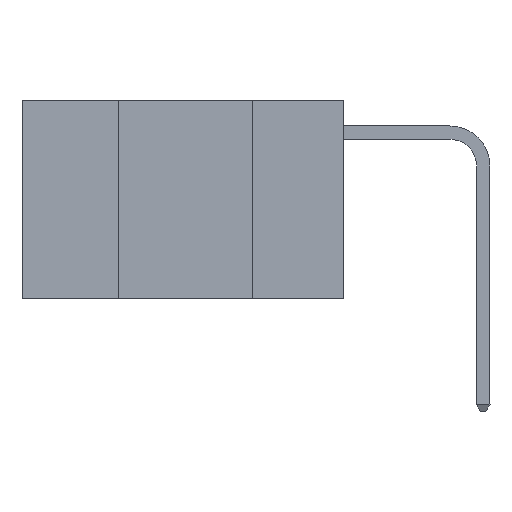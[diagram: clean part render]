
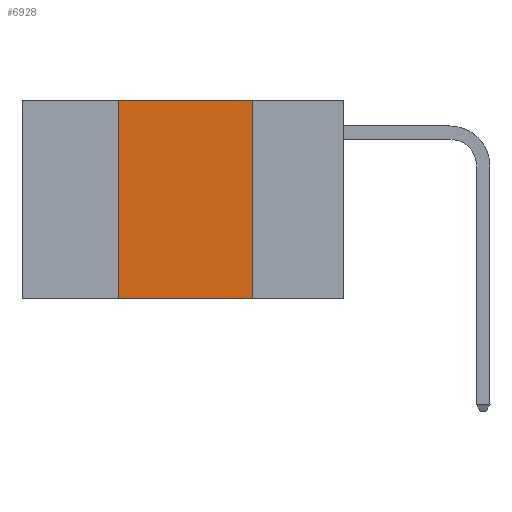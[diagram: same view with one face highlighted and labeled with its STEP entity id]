
A CAD part, left-side view. The second image highlights one B-rep face of the part: STEP entity #6928.
In plain terms, the highlighted planar face has unit normal (-1, 0, 0).
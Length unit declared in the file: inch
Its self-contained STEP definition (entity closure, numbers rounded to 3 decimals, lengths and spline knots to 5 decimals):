
#1199 = ORIENTED_EDGE ( 'NONE', *, *, #21920, .F. ) ;
#1402 = ORIENTED_EDGE ( 'NONE', *, *, #5971, .F. ) ;
#1460 = ORIENTED_EDGE ( 'NONE', *, *, #9302, .F. ) ;
#2199 = ORIENTED_EDGE ( 'NONE', *, *, #6922, .T. ) ;
#3097 = VECTOR ( 'NONE', #21161, 39.37008 ) ;
#3577 = LINE ( 'NONE', #10328, #21398 ) ;
#3950 = CARTESIAN_POINT ( 'NONE',  ( 0., 0.6, 0. ) ) ;
#4160 = DIRECTION ( 'NONE',  ( 0., 0., -1. ) ) ;
#5041 = CARTESIAN_POINT ( 'NONE',  ( 0., 0.42, -0.37 ) ) ;
#5712 = DIRECTION ( 'NONE',  ( 1., 0., 0. ) ) ;
#5971 = EDGE_CURVE ( 'NONE', #10178, #10609, #14811, .T. ) ;
#6922 = EDGE_CURVE ( 'NONE', #7887, #15546, #17515, .T. ) ;
#6928 = ADVANCED_FACE ( 'NONE', ( #20933 ), #14402, .F. ) ;
#7887 = VERTEX_POINT ( 'NONE', #5041 ) ;
#9281 = CARTESIAN_POINT ( 'NONE',  ( 0., 0.42, 0. ) ) ;
#9302 = EDGE_CURVE ( 'NONE', #7887, #10178, #3577, .T. ) ;
#9618 = CARTESIAN_POINT ( 'NONE',  ( 0., 0.17, -0.37 ) ) ;
#10169 = VECTOR ( 'NONE', #15047, 39.37008 ) ;
#10178 = VERTEX_POINT ( 'NONE', #9281 ) ;
#10328 = CARTESIAN_POINT ( 'NONE',  ( 0., 0.42, 0. ) ) ;
#10609 = VERTEX_POINT ( 'NONE', #20652 ) ;
#11359 = EDGE_LOOP ( 'NONE', ( #1199, #1402, #1460, #2199 ) ) ;
#11980 = DIRECTION ( 'NONE',  ( 0., 0., 1. ) ) ;
#12449 = LINE ( 'NONE', #14594, #21565 ) ;
#14402 = PLANE ( 'NONE',  #22063 ) ;
#14594 = CARTESIAN_POINT ( 'NONE',  ( 0., 0.17, 0. ) ) ;
#14811 = LINE ( 'NONE', #16700, #10169 ) ;
#15047 = DIRECTION ( 'NONE',  ( 0., -1., 0. ) ) ;
#15546 = VERTEX_POINT ( 'NONE', #9618 ) ;
#16700 = CARTESIAN_POINT ( 'NONE',  ( 0., 0.6, 0. ) ) ;
#17515 = LINE ( 'NONE', #19449, #3097 ) ;
#17839 = DIRECTION ( 'NONE',  ( 0., 0., -1. ) ) ;
#19449 = CARTESIAN_POINT ( 'NONE',  ( 0., 0.6, -0.37 ) ) ;
#20652 = CARTESIAN_POINT ( 'NONE',  ( 0., 0.17, 0. ) ) ;
#20933 = FACE_OUTER_BOUND ( 'NONE', #11359, .T. ) ;
#21161 = DIRECTION ( 'NONE',  ( 0., -1., 0. ) ) ;
#21398 = VECTOR ( 'NONE', #11980, 39.37008 ) ;
#21565 = VECTOR ( 'NONE', #4160, 39.37008 ) ;
#21920 = EDGE_CURVE ( 'NONE', #10609, #15546, #12449, .T. ) ;
#22063 = AXIS2_PLACEMENT_3D ( 'NONE', #3950, #5712, #17839 ) ;
